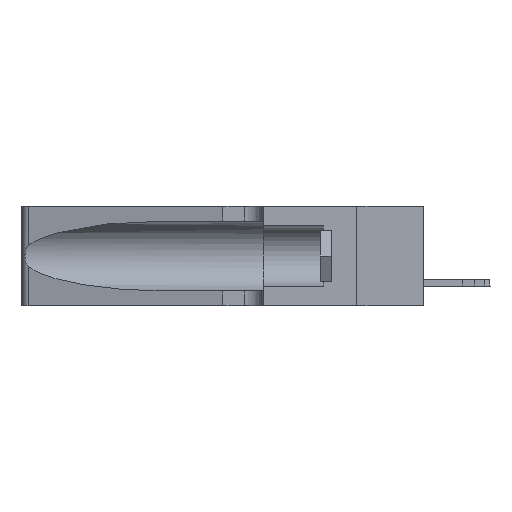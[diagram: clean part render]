
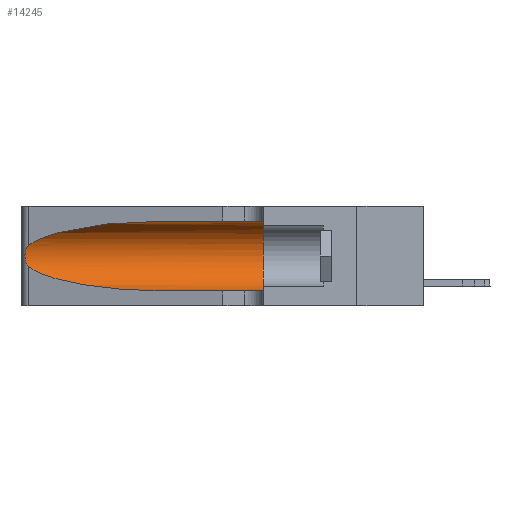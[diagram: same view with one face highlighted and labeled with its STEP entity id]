
A CAD part, left-side view. The second image highlights one B-rep face of the part: STEP entity #14245.
In plain terms, the highlighted cylindrical face has radius 3.308 mm (diameter 6.617 mm), a partial arc.
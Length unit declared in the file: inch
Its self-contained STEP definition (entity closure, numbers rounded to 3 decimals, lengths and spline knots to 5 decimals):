
#317 = CARTESIAN_POINT ( 'NONE',  ( 0.1305, 0.72297, 0.31525 ) ) ;
#708 =( BOUNDED_CURVE ( )  B_SPLINE_CURVE ( 3, ( #14414, #5851, #25734, #25640 ),
 .UNSPECIFIED., .F., .T. ) 
 B_SPLINE_CURVE_WITH_KNOTS ( ( 4, 4 ),
 ( 3.44316, 4.71239 ),
 .UNSPECIFIED. ) 
 CURVE ( )  GEOMETRIC_REPRESENTATION_ITEM ( )  RATIONAL_B_SPLINE_CURVE ( ( 1., 0.87, 0.87, 1. ) ) 
 REPRESENTATION_ITEM ( '' )  );
#1662 = CARTESIAN_POINT ( 'NONE',  ( 0.26017, 1.23833, 0.17102 ) ) ;
#1763 = VERTEX_POINT ( 'NONE', #13232 ) ;
#1856 = CARTESIAN_POINT ( 'NONE',  ( 0.26075, 1.23896, 0.178 ) ) ;
#1946 = CARTESIAN_POINT ( 'NONE',  ( 0.25787, 1.23484, 0.2124 ) ) ;
#3202 = DIRECTION ( 'NONE',  ( 0., 0., 1. ) ) ;
#3394 = ORIENTED_EDGE ( 'NONE', *, *, #5834, .F. ) ;
#4026 = CARTESIAN_POINT ( 'NONE',  ( 0.25854, 1.2359, 0.20912 ) ) ;
#4075 = FACE_OUTER_BOUND ( 'NONE', #7532, .T. ) ;
#4117 = CARTESIAN_POINT ( 'NONE',  ( 0.25789, 1.23486, 0.15765 ) ) ;
#4452 = DIRECTION ( 'NONE',  ( 0., -1., 0. ) ) ;
#5266 = VERTEX_POINT ( 'NONE', #18774 ) ;
#5280 = CARTESIAN_POINT ( 'NONE',  ( 0.2373, 1.15595, 0.28018 ) ) ;
#5379 = CARTESIAN_POINT ( 'NONE',  ( 0.25487, 1.22718, 0.22369 ) ) ;
#5531 =( BOUNDED_CURVE ( )  B_SPLINE_CURVE ( 3, ( #317, #7010, #5280, #5379 ),
 .UNSPECIFIED., .F., .F. ) 
 B_SPLINE_CURVE_WITH_KNOTS ( ( 4, 4 ),
 ( 1.5708, 2.84003 ),
 .UNSPECIFIED. ) 
 CURVE ( )  GEOMETRIC_REPRESENTATION_ITEM ( )  RATIONAL_B_SPLINE_CURVE ( ( 1., 0.87, 0.87, 1. ) ) 
 REPRESENTATION_ITEM ( '' )  );
#5799 = CYLINDRICAL_SURFACE ( 'NONE', #27664, 0.13025 ) ;
#5834 = EDGE_CURVE ( 'NONE', #16901, #19717, #15174, .T. ) ;
#5851 = CARTESIAN_POINT ( 'NONE',  ( 0.2373, 1.15595, 0.08982 ) ) ;
#6014 = DIRECTION ( 'NONE',  ( 0., -1., 0. ) ) ;
#6450 = DIRECTION ( 'NONE',  ( 0., 0., -1. ) ) ;
#7010 = CARTESIAN_POINT ( 'NONE',  ( 0.18966, 0.96281, 0.31525 ) ) ;
#7532 = EDGE_LOOP ( 'NONE', ( #18557, #16194, #9961, #9633, #3394, #23899 ) ) ;
#7611 = LINE ( 'NONE', #17285, #7954 ) ;
#7954 = VECTOR ( 'NONE', #6014, 39.37008 ) ;
#8266 = CARTESIAN_POINT ( 'NONE',  ( 0.25487, 1.22718, 0.22369 ) ) ;
#8355 = CARTESIAN_POINT ( 'NONE',  ( 0.25487, 1.22718, 0.14631 ) ) ;
#8547 = CARTESIAN_POINT ( 'NONE',  ( 0.25555, 1.22993, 0.14849 ) ) ;
#9324 = CARTESIAN_POINT ( 'NONE',  ( 0.1305, 0.35, 0.05475 ) ) ;
#9633 = ORIENTED_EDGE ( 'NONE', *, *, #20206, .T. ) ;
#9961 = ORIENTED_EDGE ( 'NONE', *, *, #12550, .T. ) ;
#10720 = CARTESIAN_POINT ( 'NONE',  ( 0.26075, 1.23896, 0.19203 ) ) ;
#11432 = CARTESIAN_POINT ( 'NONE',  ( 0.1305, 1.61858, 0.05475 ) ) ;
#11653 = CARTESIAN_POINT ( 'NONE',  ( 0.1305, 0.35, 0.31525 ) ) ;
#12039 = EDGE_CURVE ( 'NONE', #22299, #16901, #7611, .T. ) ;
#12550 = EDGE_CURVE ( 'NONE', #1763, #20921, #708, .T. ) ;
#12761 = CARTESIAN_POINT ( 'NONE',  ( 0.26018, 1.23835, 0.19895 ) ) ;
#13232 = CARTESIAN_POINT ( 'NONE',  ( 0.25487, 1.22718, 0.14631 ) ) ;
#14245 = ADVANCED_FACE ( 'NONE', ( #4075 ), #5799, .F. ) ;
#14414 = CARTESIAN_POINT ( 'NONE',  ( 0.25487, 1.22718, 0.14631 ) ) ;
#14563 = LINE ( 'NONE', #11432, #17666 ) ;
#14980 = CARTESIAN_POINT ( 'NONE',  ( 0.25555, 1.22994, 0.2215 ) ) ;
#15165 = CARTESIAN_POINT ( 'NONE',  ( 0.25639, 1.23186, 0.15144 ) ) ;
#15174 = CIRCLE ( 'NONE', #23422, 0.13025 ) ;
#16194 = ORIENTED_EDGE ( 'NONE', *, *, #19305, .T. ) ;
#16620 = CARTESIAN_POINT ( 'NONE',  ( 0.1305, 0.72297, 0.31525 ) ) ;
#16901 = VERTEX_POINT ( 'NONE', #11653 ) ;
#17285 = CARTESIAN_POINT ( 'NONE',  ( 0.1305, 1.61858, 0.31525 ) ) ;
#17303 = CARTESIAN_POINT ( 'NONE',  ( 0.25639, 1.23184, 0.21858 ) ) ;
#17578 = CARTESIAN_POINT ( 'NONE',  ( 0.25856, 1.23593, 0.16098 ) ) ;
#17666 = VECTOR ( 'NONE', #4452, 39.37008 ) ;
#18557 = ORIENTED_EDGE ( 'NONE', *, *, #25217, .T. ) ;
#18774 = CARTESIAN_POINT ( 'NONE',  ( 0.25487, 1.22718, 0.22369 ) ) ;
#19305 = EDGE_CURVE ( 'NONE', #5266, #1763, #26526, .T. ) ;
#19717 = VERTEX_POINT ( 'NONE', #9324 ) ;
#20139 = DIRECTION ( 'NONE',  ( 0., -1., 0. ) ) ;
#20206 = EDGE_CURVE ( 'NONE', #20921, #19717, #14563, .T. ) ;
#20921 = VERTEX_POINT ( 'NONE', #27365 ) ;
#21043 = DIRECTION ( 'NONE',  ( 0., 1., 0. ) ) ;
#22299 = VERTEX_POINT ( 'NONE', #16620 ) ;
#23422 = AXIS2_PLACEMENT_3D ( 'NONE', #25309, #21043, #3202 ) ;
#23899 = ORIENTED_EDGE ( 'NONE', *, *, #12039, .F. ) ;
#24404 = CARTESIAN_POINT ( 'NONE',  ( 0.1305, 1.61858, 0.185 ) ) ;
#25217 = EDGE_CURVE ( 'NONE', #22299, #5266, #5531, .T. ) ;
#25309 = CARTESIAN_POINT ( 'NONE',  ( 0.1305, 0.35, 0.185 ) ) ;
#25640 = CARTESIAN_POINT ( 'NONE',  ( 0.1305, 0.72297, 0.05475 ) ) ;
#25734 = CARTESIAN_POINT ( 'NONE',  ( 0.18966, 0.96281, 0.05475 ) ) ;
#26526 = B_SPLINE_CURVE_WITH_KNOTS ( 'NONE', 3,
 ( #8266, #14980, #17303, #1946, #4026, #12761, #10720, #1856, #1662, #17578, #4117, #15165, #8547, #8355 ),
 .UNSPECIFIED., .F., .F.,
 ( 4, 2, 2, 2, 2, 2, 4 ),
 ( 0., 0.00027, 0.00053, 0.00107, 0.0016, 0.00187, 0.00214 ),
 .UNSPECIFIED. ) ;
#27365 = CARTESIAN_POINT ( 'NONE',  ( 0.1305, 0.72297, 0.05475 ) ) ;
#27664 = AXIS2_PLACEMENT_3D ( 'NONE', #24404, #20139, #6450 ) ;
